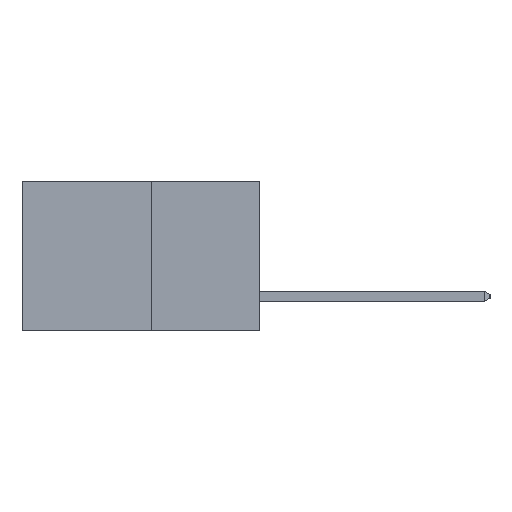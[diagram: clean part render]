
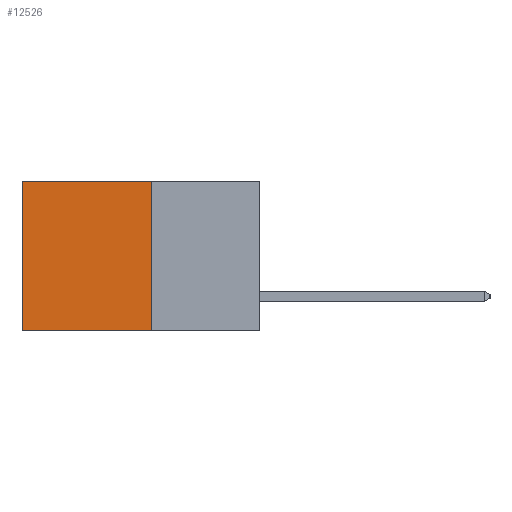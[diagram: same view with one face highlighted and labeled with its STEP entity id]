
A CAD part, left-side view. The second image highlights one B-rep face of the part: STEP entity #12526.
In plain terms, the highlighted planar face has unit normal (-1, 0, 0).
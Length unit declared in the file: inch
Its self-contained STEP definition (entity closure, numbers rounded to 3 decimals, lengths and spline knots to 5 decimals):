
#27 = EDGE_CURVE ( 'NONE', #11622, #6928, #3103, .T. ) ;
#108 = EDGE_CURVE ( 'NONE', #6502, #11622, #1424, .T. ) ;
#150 = DIRECTION ( 'NONE',  ( 0., 1., 0. ) ) ;
#539 = CARTESIAN_POINT ( 'NONE',  ( 0.277, 0.27, -0.37 ) ) ;
#576 = DIRECTION ( 'NONE',  ( 0., 0., -1. ) ) ;
#1056 = ORIENTED_EDGE ( 'NONE', *, *, #4359, .T. ) ;
#1424 = LINE ( 'NONE', #11709, #7775 ) ;
#1685 = VERTEX_POINT ( 'NONE', #3476 ) ;
#1883 = PLANE ( 'NONE',  #3214 ) ;
#2234 = CARTESIAN_POINT ( 'NONE',  ( 0.277, 0.59, -0.37 ) ) ;
#2364 = ORIENTED_EDGE ( 'NONE', *, *, #108, .F. ) ;
#2871 = ORIENTED_EDGE ( 'NONE', *, *, #4461, .T. ) ;
#3103 = LINE ( 'NONE', #539, #6503 ) ;
#3214 = AXIS2_PLACEMENT_3D ( 'NONE', #11711, #4532, #12878 ) ;
#3476 = CARTESIAN_POINT ( 'NONE',  ( 0.277, 0.59, 0. ) ) ;
#4175 = LINE ( 'NONE', #14220, #13351 ) ;
#4359 = EDGE_CURVE ( 'NONE', #1685, #6928, #4175, .T. ) ;
#4461 = EDGE_CURVE ( 'NONE', #6502, #1685, #11139, .T. ) ;
#4532 = DIRECTION ( 'NONE',  ( 1., 0., 0. ) ) ;
#4752 = VECTOR ( 'NONE', #150, 39.37008 ) ;
#5547 = CARTESIAN_POINT ( 'NONE',  ( 0.277, 0.27, 0. ) ) ;
#6502 = VERTEX_POINT ( 'NONE', #5547 ) ;
#6503 = VECTOR ( 'NONE', #11541, 39.37008 ) ;
#6928 = VERTEX_POINT ( 'NONE', #2234 ) ;
#7775 = VECTOR ( 'NONE', #12996, 39.37008 ) ;
#10546 = CARTESIAN_POINT ( 'NONE',  ( 0.277, 0.27, -0.37 ) ) ;
#11139 = LINE ( 'NONE', #12660, #4752 ) ;
#11541 = DIRECTION ( 'NONE',  ( 0., 1., 0. ) ) ;
#11622 = VERTEX_POINT ( 'NONE', #10546 ) ;
#11709 = CARTESIAN_POINT ( 'NONE',  ( 0.277, 0.27, -0.37 ) ) ;
#11711 = CARTESIAN_POINT ( 'NONE',  ( 0.277, 0.27, -0.37 ) ) ;
#12526 = ADVANCED_FACE ( 'NONE', ( #15711 ), #1883, .F. ) ;
#12660 = CARTESIAN_POINT ( 'NONE',  ( 0.277, 0.27, 0. ) ) ;
#12878 = DIRECTION ( 'NONE',  ( 0., 0., -1. ) ) ;
#12996 = DIRECTION ( 'NONE',  ( 0., 0., -1. ) ) ;
#13267 = ORIENTED_EDGE ( 'NONE', *, *, #27, .F. ) ;
#13351 = VECTOR ( 'NONE', #576, 39.37008 ) ;
#14220 = CARTESIAN_POINT ( 'NONE',  ( 0.277, 0.59, -0.37 ) ) ;
#14221 = EDGE_LOOP ( 'NONE', ( #1056, #13267, #2364, #2871 ) ) ;
#15711 = FACE_OUTER_BOUND ( 'NONE', #14221, .T. ) ;
